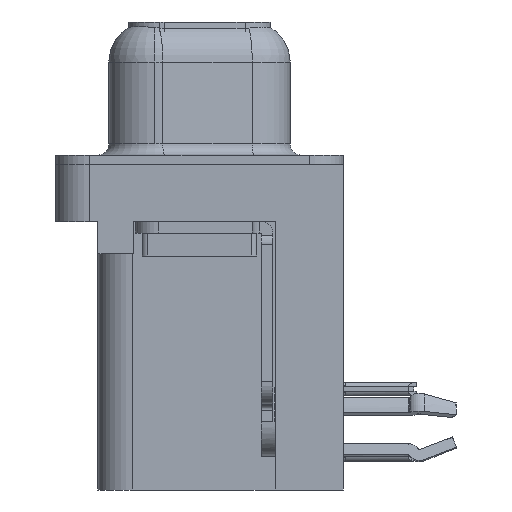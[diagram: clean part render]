
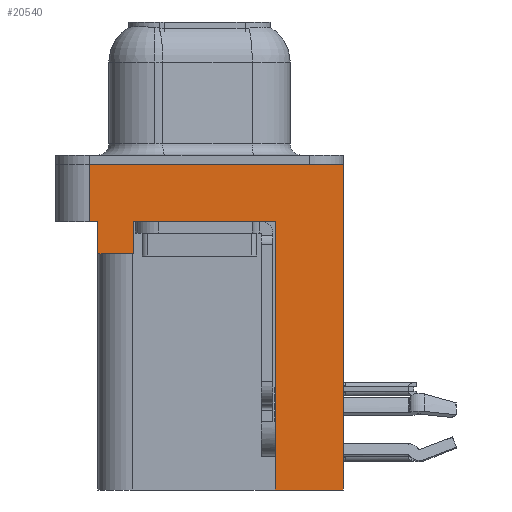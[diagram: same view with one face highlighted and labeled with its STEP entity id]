
A CAD part, left-side view. The second image highlights one B-rep face of the part: STEP entity #20540.
In plain terms, the highlighted planar face has unit normal (-1, 0, 0).
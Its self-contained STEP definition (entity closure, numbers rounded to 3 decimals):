
#222 = CARTESIAN_POINT ( 'NONE',  ( -3., -6.275, -2.5 ) ) ;
#303 = CARTESIAN_POINT ( 'NONE',  ( -3., -6.275, 0. ) ) ;
#329 = VERTEX_POINT ( 'NONE', #17004 ) ;
#365 = AXIS2_PLACEMENT_3D ( 'NONE', #28076, #32727, #5016 ) ;
#495 = DIRECTION ( 'NONE',  ( 0., 0., 1. ) ) ;
#736 = ORIENTED_EDGE ( 'NONE', *, *, #31246, .T. ) ;
#854 = ORIENTED_EDGE ( 'NONE', *, *, #20379, .F. ) ;
#986 = VERTEX_POINT ( 'NONE', #21087 ) ;
#1291 = EDGE_CURVE ( 'NONE', #986, #22265, #25057, .T. ) ;
#2210 = VERTEX_POINT ( 'NONE', #21584 ) ;
#2349 = VECTOR ( 'NONE', #8885, 1000. ) ;
#2358 = CARTESIAN_POINT ( 'NONE',  ( -3., 4.425, -3.9 ) ) ;
#4059 = ORIENTED_EDGE ( 'NONE', *, *, #18317, .T. ) ;
#5016 = DIRECTION ( 'NONE',  ( 0., 0., 1. ) ) ;
#5343 = VECTOR ( 'NONE', #20430, 1000. ) ;
#5667 = CARTESIAN_POINT ( 'NONE',  ( -3., -6.275, -2.5 ) ) ;
#5920 = EDGE_CURVE ( 'NONE', #18612, #22265, #22931, .T. ) ;
#6074 = VECTOR ( 'NONE', #495, 1000. ) ;
#6930 = ORIENTED_EDGE ( 'NONE', *, *, #23918, .F. ) ;
#7098 = CARTESIAN_POINT ( 'NONE',  ( -3., 4.425, -2.5 ) ) ;
#7252 = EDGE_CURVE ( 'NONE', #24799, #19711, #12346, .T. ) ;
#8885 = DIRECTION ( 'NONE',  ( 0., 0., 1. ) ) ;
#10162 = CARTESIAN_POINT ( 'NONE',  ( -3., -3.295, -14.2 ) ) ;
#10345 = ORIENTED_EDGE ( 'NONE', *, *, #1291, .F. ) ;
#11668 = EDGE_CURVE ( 'NONE', #31325, #329, #31638, .T. ) ;
#11713 = EDGE_LOOP ( 'NONE', ( #16441, #22104, #24622, #10345, #6930, #16910, #736, #17153, #854, #4059 ) ) ;
#12346 = LINE ( 'NONE', #29459, #12598 ) ;
#12494 = VECTOR ( 'NONE', #16640, 1000. ) ;
#12592 = CARTESIAN_POINT ( 'NONE',  ( -3., 4.775, -2.5 ) ) ;
#12598 = VECTOR ( 'NONE', #22488, 1000. ) ;
#12816 = LINE ( 'NONE', #10162, #24981 ) ;
#12921 = DIRECTION ( 'NONE',  ( 0., 0., 1. ) ) ;
#13014 = CARTESIAN_POINT ( 'NONE',  ( -3., 4.425, -3.9 ) ) ;
#13134 = DIRECTION ( 'NONE',  ( 0., 0., 1. ) ) ;
#13139 = EDGE_CURVE ( 'NONE', #30552, #2210, #12816, .T. ) ;
#13871 = VECTOR ( 'NONE', #15789, 1000. ) ;
#14178 = CARTESIAN_POINT ( 'NONE',  ( -3., -3.295, -14.2 ) ) ;
#14292 = LINE ( 'NONE', #29417, #12494 ) ;
#15789 = DIRECTION ( 'NONE',  ( 0., -1., 0. ) ) ;
#16441 = ORIENTED_EDGE ( 'NONE', *, *, #7252, .F. ) ;
#16640 = DIRECTION ( 'NONE',  ( 0., 1., 0. ) ) ;
#16910 = ORIENTED_EDGE ( 'NONE', *, *, #11668, .T. ) ;
#17004 = CARTESIAN_POINT ( 'NONE',  ( -3., 2.895, -2.5 ) ) ;
#17153 = ORIENTED_EDGE ( 'NONE', *, *, #13139, .F. ) ;
#17326 = EDGE_CURVE ( 'NONE', #18612, #24799, #22898, .T. ) ;
#18112 = VERTEX_POINT ( 'NONE', #32180 ) ;
#18317 = EDGE_CURVE ( 'NONE', #18112, #19711, #30671, .T. ) ;
#18380 = CARTESIAN_POINT ( 'NONE',  ( -3., -6.275, -2.5 ) ) ;
#18541 = CARTESIAN_POINT ( 'NONE',  ( -3., 2.895, -3.9 ) ) ;
#18612 = VERTEX_POINT ( 'NONE', #32141 ) ;
#19711 = VERTEX_POINT ( 'NONE', #303 ) ;
#20051 = DIRECTION ( 'NONE',  ( 0., 0., 1. ) ) ;
#20379 = EDGE_CURVE ( 'NONE', #18112, #30552, #14292, .T. ) ;
#20430 = DIRECTION ( 'NONE',  ( 0., -1., 0. ) ) ;
#20540 = ADVANCED_FACE ( 'NONE', ( #25752 ), #23093, .T. ) ;
#21087 = CARTESIAN_POINT ( 'NONE',  ( -3., 4.425, -3.9 ) ) ;
#21584 = CARTESIAN_POINT ( 'NONE',  ( -3., -3.295, -2.5 ) ) ;
#22104 = ORIENTED_EDGE ( 'NONE', *, *, #17326, .F. ) ;
#22265 = VERTEX_POINT ( 'NONE', #7098 ) ;
#22488 = DIRECTION ( 'NONE',  ( 0., -1., 0. ) ) ;
#22898 = LINE ( 'NONE', #12592, #26691 ) ;
#22931 = LINE ( 'NONE', #222, #5343 ) ;
#23093 = PLANE ( 'NONE',  #365 ) ;
#23918 = EDGE_CURVE ( 'NONE', #31325, #986, #25653, .T. ) ;
#24622 = ORIENTED_EDGE ( 'NONE', *, *, #5920, .T. ) ;
#24799 = VERTEX_POINT ( 'NONE', #29319 ) ;
#24981 = VECTOR ( 'NONE', #13134, 1000. ) ;
#25057 = LINE ( 'NONE', #2358, #32458 ) ;
#25653 = LINE ( 'NONE', #13014, #30610 ) ;
#25752 = FACE_OUTER_BOUND ( 'NONE', #11713, .T. ) ;
#26691 = VECTOR ( 'NONE', #12921, 1000. ) ;
#26825 = CARTESIAN_POINT ( 'NONE',  ( -3., 2.895, -3.9 ) ) ;
#28076 = CARTESIAN_POINT ( 'NONE',  ( -3., -6.275, -2.5 ) ) ;
#28416 = LINE ( 'NONE', #5667, #13871 ) ;
#29319 = CARTESIAN_POINT ( 'NONE',  ( -3., 4.775, 0. ) ) ;
#29417 = CARTESIAN_POINT ( 'NONE',  ( -3., -3.295, -14.2 ) ) ;
#29459 = CARTESIAN_POINT ( 'NONE',  ( -3., -6.275, 0. ) ) ;
#30552 = VERTEX_POINT ( 'NONE', #14178 ) ;
#30610 = VECTOR ( 'NONE', #30787, 1000. ) ;
#30671 = LINE ( 'NONE', #18380, #6074 ) ;
#30787 = DIRECTION ( 'NONE',  ( 0., 1., 0. ) ) ;
#31246 = EDGE_CURVE ( 'NONE', #329, #2210, #28416, .T. ) ;
#31325 = VERTEX_POINT ( 'NONE', #18541 ) ;
#31638 = LINE ( 'NONE', #26825, #2349 ) ;
#32141 = CARTESIAN_POINT ( 'NONE',  ( -3., 4.775, -2.5 ) ) ;
#32180 = CARTESIAN_POINT ( 'NONE',  ( -3., -6.275, -14.2 ) ) ;
#32458 = VECTOR ( 'NONE', #20051, 1000. ) ;
#32727 = DIRECTION ( 'NONE',  ( -1., 0., 0. ) ) ;
